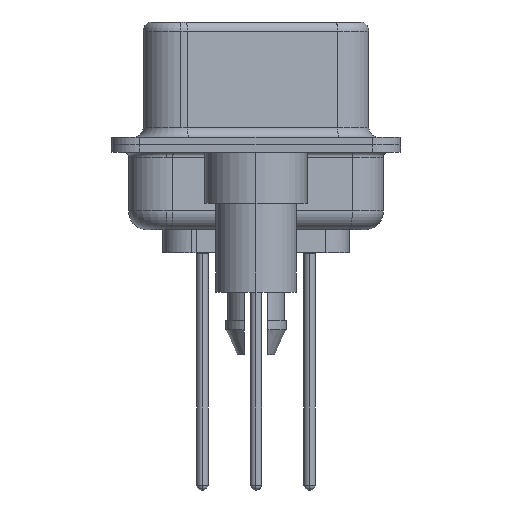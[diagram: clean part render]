
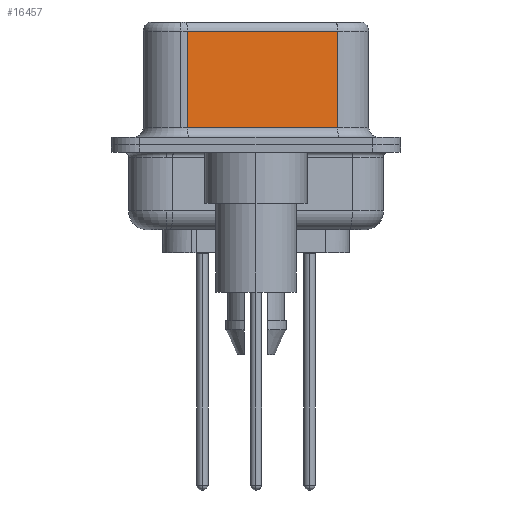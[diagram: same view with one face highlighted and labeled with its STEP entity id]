
A CAD part, left-side view. The second image highlights one B-rep face of the part: STEP entity #16457.
In plain terms, the highlighted planar face has unit normal (-0.985, -0.174, 0).
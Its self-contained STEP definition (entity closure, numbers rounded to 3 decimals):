
#694 = DIRECTION ( 'NONE',  ( 0., 0., -1. ) ) ;
#965 = ORIENTED_EDGE ( 'NONE', *, *, #17419, .F. ) ;
#2461 = CARTESIAN_POINT ( 'NONE',  ( 5.132, -4.322, 6.52 ) ) ;
#3336 = VERTEX_POINT ( 'NONE', #19944 ) ;
#4786 = ORIENTED_EDGE ( 'NONE', *, *, #19192, .T. ) ;
#6582 = CARTESIAN_POINT ( 'NONE',  ( 5.132, -4.322, 0.9 ) ) ;
#6840 = EDGE_CURVE ( 'NONE', #26583, #8981, #19378, .T. ) ;
#6858 = CARTESIAN_POINT ( 'NONE',  ( 3.73, 3.628, 0.9 ) ) ;
#6899 = PLANE ( 'NONE',  #12306 ) ;
#7624 = ORIENTED_EDGE ( 'NONE', *, *, #23715, .T. ) ;
#8026 = CARTESIAN_POINT ( 'NONE',  ( 3.73, 3.628, 6.52 ) ) ;
#8981 = VERTEX_POINT ( 'NONE', #6858 ) ;
#9481 = DIRECTION ( 'NONE',  ( 0.985, 0.174, 0. ) ) ;
#11445 = LINE ( 'NONE', #6582, #17026 ) ;
#12306 = AXIS2_PLACEMENT_3D ( 'NONE', #2461, #9481, #26028 ) ;
#14512 = VERTEX_POINT ( 'NONE', #22722 ) ;
#15924 = DIRECTION ( 'NONE',  ( 0.174, -0.985, 0. ) ) ;
#16247 = FACE_OUTER_BOUND ( 'NONE', #26610, .T. ) ;
#16293 = CARTESIAN_POINT ( 'NONE',  ( 5.132, -4.322, 6.02 ) ) ;
#16457 = ADVANCED_FACE ( 'NONE', ( #16247 ), #6899, .F. ) ;
#17026 = VECTOR ( 'NONE', #15924, 1000. ) ;
#17419 = EDGE_CURVE ( 'NONE', #14512, #3336, #20621, .T. ) ;
#17561 = VECTOR ( 'NONE', #694, 1000. ) ;
#19192 = EDGE_CURVE ( 'NONE', #14512, #26583, #23200, .T. ) ;
#19378 = LINE ( 'NONE', #8026, #17561 ) ;
#19486 = ORIENTED_EDGE ( 'NONE', *, *, #6840, .T. ) ;
#19944 = CARTESIAN_POINT ( 'NONE',  ( 5.132, -4.322, 0.9 ) ) ;
#20621 = LINE ( 'NONE', #29968, #26080 ) ;
#21180 = DIRECTION ( 'NONE',  ( -0.174, 0.985, 0. ) ) ;
#22722 = CARTESIAN_POINT ( 'NONE',  ( 5.132, -4.322, 6.02 ) ) ;
#23200 = LINE ( 'NONE', #16293, #23664 ) ;
#23664 = VECTOR ( 'NONE', #21180, 1000. ) ;
#23715 = EDGE_CURVE ( 'NONE', #8981, #3336, #11445, .T. ) ;
#25376 = DIRECTION ( 'NONE',  ( 0., 0., -1. ) ) ;
#26028 = DIRECTION ( 'NONE',  ( -0.174, 0.985, 0. ) ) ;
#26080 = VECTOR ( 'NONE', #25376, 1000. ) ;
#26583 = VERTEX_POINT ( 'NONE', #28198 ) ;
#26610 = EDGE_LOOP ( 'NONE', ( #965, #4786, #19486, #7624 ) ) ;
#28198 = CARTESIAN_POINT ( 'NONE',  ( 3.73, 3.628, 6.02 ) ) ;
#29968 = CARTESIAN_POINT ( 'NONE',  ( 5.132, -4.322, 6.52 ) ) ;
